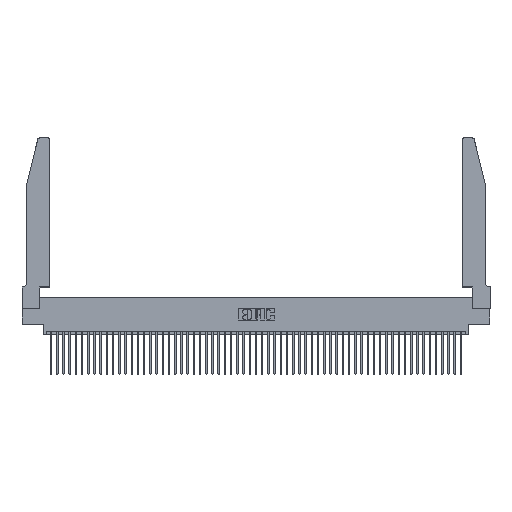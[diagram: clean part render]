
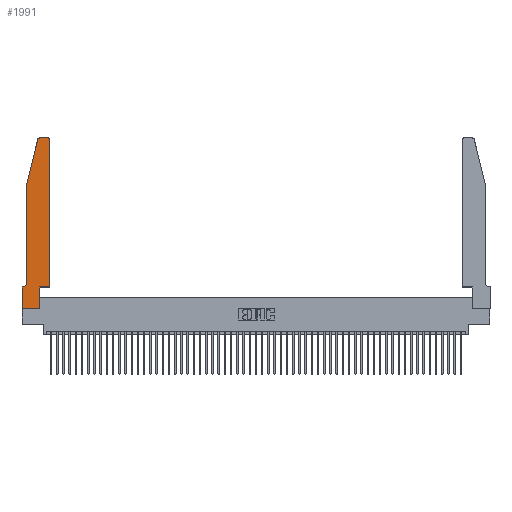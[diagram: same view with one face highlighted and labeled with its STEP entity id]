
A CAD part, top view. The second image highlights one B-rep face of the part: STEP entity #1991.
In plain terms, the highlighted planar face has unit normal (0, 0, 1).
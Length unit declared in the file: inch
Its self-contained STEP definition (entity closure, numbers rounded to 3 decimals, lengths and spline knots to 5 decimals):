
#371 = VERTEX_POINT ( 'NONE', #52718 ) ;
#665 = DIRECTION ( 'NONE',  ( 0., 0., 1. ) ) ;
#1611 = ORIENTED_EDGE ( 'NONE', *, *, #6395, .T. ) ;
#1833 = CARTESIAN_POINT ( 'NONE',  ( 0.4505, 2.72, 0.37 ) ) ;
#1884 = DIRECTION ( 'NONE',  ( 0., -1., 0. ) ) ;
#1991 = ADVANCED_FACE ( 'NONE', ( #21943 ), #21525, .T. ) ;
#2084 = VECTOR ( 'NONE', #26790, 39.37008 ) ;
#2314 = EDGE_CURVE ( 'NONE', #29373, #42657, #33009, .T. ) ;
#3497 = CARTESIAN_POINT ( 'NONE',  ( 0.0055, 0.42, 0.37 ) ) ;
#3612 = CARTESIAN_POINT ( 'NONE',  ( 0., 0., 0.37 ) ) ;
#4301 = VERTEX_POINT ( 'NONE', #50310 ) ;
#5514 = AXIS2_PLACEMENT_3D ( 'NONE', #13856, #43081, #51312 ) ;
#5885 = AXIS2_PLACEMENT_3D ( 'NONE', #49637, #8313, #29193 ) ;
#6395 = EDGE_CURVE ( 'NONE', #4301, #37584, #19648, .T. ) ;
#6744 = CIRCLE ( 'NONE', #5885, 0.03 ) ;
#7125 = EDGE_CURVE ( 'NONE', #31147, #17928, #8435, .T. ) ;
#8038 = CARTESIAN_POINT ( 'NONE',  ( 0.284, 2.75, 0.37 ) ) ;
#8313 = DIRECTION ( 'NONE',  ( 0., 0., 1. ) ) ;
#8435 = LINE ( 'NONE', #26455, #36580 ) ;
#8854 = CARTESIAN_POINT ( 'NONE',  ( 0.0755, 2., 0.37 ) ) ;
#9084 = VERTEX_POINT ( 'NONE', #14801 ) ;
#10974 = ORIENTED_EDGE ( 'NONE', *, *, #46758, .T. ) ;
#11453 = CARTESIAN_POINT ( 'NONE',  ( 0.0755, 2., 0.37 ) ) ;
#12211 = EDGE_CURVE ( 'NONE', #9084, #17932, #51008, .T. ) ;
#13390 = EDGE_CURVE ( 'NONE', #37584, #16904, #32595, .T. ) ;
#13509 = ORIENTED_EDGE ( 'NONE', *, *, #13390, .T. ) ;
#13550 = LINE ( 'NONE', #45779, #29234 ) ;
#13856 = CARTESIAN_POINT ( 'NONE',  ( 0.284, 2.72, 0.37 ) ) ;
#14271 = ORIENTED_EDGE ( 'NONE', *, *, #12211, .T. ) ;
#14524 = VECTOR ( 'NONE', #28611, 39.37008 ) ;
#14801 = CARTESIAN_POINT ( 'NONE',  ( 0.0055, 0.35, 0.37 ) ) ;
#15091 = VECTOR ( 'NONE', #16419, 39.37008 ) ;
#15588 = VERTEX_POINT ( 'NONE', #38577 ) ;
#15670 = CARTESIAN_POINT ( 'NONE',  ( 0.4205, 2.75, 0.37 ) ) ;
#16419 = DIRECTION ( 'NONE',  ( 1., 0., 0. ) ) ;
#16428 = VECTOR ( 'NONE', #1884, 39.37008 ) ;
#16904 = VERTEX_POINT ( 'NONE', #47581 ) ;
#17928 = VERTEX_POINT ( 'NONE', #24048 ) ;
#17932 = VERTEX_POINT ( 'NONE', #27929 ) ;
#18575 = CARTESIAN_POINT ( 'NONE',  ( 0.0755, 0.35, 0.37 ) ) ;
#19648 = LINE ( 'NONE', #3612, #15091 ) ;
#19733 = CARTESIAN_POINT ( 'NONE',  ( 0.2865, 0., 0.37 ) ) ;
#21005 = EDGE_LOOP ( 'NONE', ( #46858, #48143, #28346, #28742, #32800, #14271, #38898, #1611, #13509, #22802, #46341, #10974 ) ) ;
#21525 = PLANE ( 'NONE',  #49095 ) ;
#21943 = FACE_OUTER_BOUND ( 'NONE', #21005, .T. ) ;
#22062 = CARTESIAN_POINT ( 'NONE',  ( 0., 0.35, 0.37 ) ) ;
#22802 = ORIENTED_EDGE ( 'NONE', *, *, #38465, .T. ) ;
#23965 = VERTEX_POINT ( 'NONE', #1833 ) ;
#24048 = CARTESIAN_POINT ( 'NONE',  ( 0.0755, 0.42, 0.37 ) ) ;
#24708 = EDGE_CURVE ( 'NONE', #15588, #23965, #53706, .T. ) ;
#25255 = EDGE_CURVE ( 'NONE', #17932, #4301, #47117, .T. ) ;
#25888 = DIRECTION ( 'NONE',  ( 1., 0., 0. ) ) ;
#26049 = DIRECTION ( 'NONE',  ( -1., 0., 0. ) ) ;
#26455 = CARTESIAN_POINT ( 'NONE',  ( 0.0755, 2., 0.37 ) ) ;
#26790 = DIRECTION ( 'NONE',  ( -1., 0., 0. ) ) ;
#26920 = CARTESIAN_POINT ( 'NONE',  ( 0., 0., 0.37 ) ) ;
#27929 = CARTESIAN_POINT ( 'NONE',  ( 0., 0.35, 0.37 ) ) ;
#28346 = ORIENTED_EDGE ( 'NONE', *, *, #29356, .T. ) ;
#28442 = CARTESIAN_POINT ( 'NONE',  ( 0.4505, 0.35, 0.37 ) ) ;
#28611 = DIRECTION ( 'NONE',  ( 0., 1., 0. ) ) ;
#28742 = ORIENTED_EDGE ( 'NONE', *, *, #7125, .T. ) ;
#29193 = DIRECTION ( 'NONE',  ( 1., 0., 0. ) ) ;
#29234 = VECTOR ( 'NONE', #38139, 39.37008 ) ;
#29356 = EDGE_CURVE ( 'NONE', #371, #31147, #42398, .T. ) ;
#29373 = VERTEX_POINT ( 'NONE', #15670 ) ;
#30569 = DIRECTION ( 'NONE',  ( 0., 1., 0. ) ) ;
#31147 = VERTEX_POINT ( 'NONE', #8854 ) ;
#31318 = VECTOR ( 'NONE', #48359, 39.37008 ) ;
#32595 = LINE ( 'NONE', #34596, #41067 ) ;
#32800 = ORIENTED_EDGE ( 'NONE', *, *, #53807, .T. ) ;
#33009 = LINE ( 'NONE', #53330, #50647 ) ;
#33745 = DIRECTION ( 'NONE',  ( 0., -1., 0. ) ) ;
#34596 = CARTESIAN_POINT ( 'NONE',  ( 0.2865, 0.35, 0.37 ) ) ;
#36580 = VECTOR ( 'NONE', #33745, 39.37008 ) ;
#37584 = VERTEX_POINT ( 'NONE', #19733 ) ;
#38139 = DIRECTION ( 'NONE',  ( 1., 0., 0. ) ) ;
#38465 = EDGE_CURVE ( 'NONE', #16904, #15588, #13550, .T. ) ;
#38577 = CARTESIAN_POINT ( 'NONE',  ( 0.4505, 0.35, 0.37 ) ) ;
#38898 = ORIENTED_EDGE ( 'NONE', *, *, #25255, .T. ) ;
#39125 = DIRECTION ( 'NONE',  ( -1., 0., 0. ) ) ;
#39341 = EDGE_CURVE ( 'NONE', #42657, #371, #50075, .T. ) ;
#41067 = VECTOR ( 'NONE', #30569, 39.37008 ) ;
#41761 = CIRCLE ( 'NONE', #44634, 0.07 ) ;
#42398 = LINE ( 'NONE', #11453, #31318 ) ;
#42657 = VERTEX_POINT ( 'NONE', #8038 ) ;
#43081 = DIRECTION ( 'NONE',  ( 0., 0., 1. ) ) ;
#44634 = AXIS2_PLACEMENT_3D ( 'NONE', #3497, #51066, #26049 ) ;
#45779 = CARTESIAN_POINT ( 'NONE',  ( 0.4505, 0.35, 0.37 ) ) ;
#46341 = ORIENTED_EDGE ( 'NONE', *, *, #24708, .T. ) ;
#46758 = EDGE_CURVE ( 'NONE', #23965, #29373, #6744, .T. ) ;
#46858 = ORIENTED_EDGE ( 'NONE', *, *, #2314, .T. ) ;
#47117 = LINE ( 'NONE', #26920, #16428 ) ;
#47581 = CARTESIAN_POINT ( 'NONE',  ( 0.2865, 0.35, 0.37 ) ) ;
#48143 = ORIENTED_EDGE ( 'NONE', *, *, #39341, .T. ) ;
#48359 = DIRECTION ( 'NONE',  ( -0.239, -0.971, 0. ) ) ;
#49095 = AXIS2_PLACEMENT_3D ( 'NONE', #22062, #665, #25888 ) ;
#49637 = CARTESIAN_POINT ( 'NONE',  ( 0.4205, 2.72, 0.37 ) ) ;
#50075 = CIRCLE ( 'NONE', #5514, 0.03 ) ;
#50310 = CARTESIAN_POINT ( 'NONE',  ( 0., 0., 0.37 ) ) ;
#50647 = VECTOR ( 'NONE', #39125, 39.37008 ) ;
#51008 = LINE ( 'NONE', #18575, #2084 ) ;
#51066 = DIRECTION ( 'NONE',  ( 0., 0., -1. ) ) ;
#51312 = DIRECTION ( 'NONE',  ( 1., 0., 0. ) ) ;
#52718 = CARTESIAN_POINT ( 'NONE',  ( 0.25487, 2.72718, 0.37 ) ) ;
#53330 = CARTESIAN_POINT ( 'NONE',  ( 0.2605, 2.75, 0.37 ) ) ;
#53706 = LINE ( 'NONE', #28442, #14524 ) ;
#53807 = EDGE_CURVE ( 'NONE', #17928, #9084, #41761, .T. ) ;
